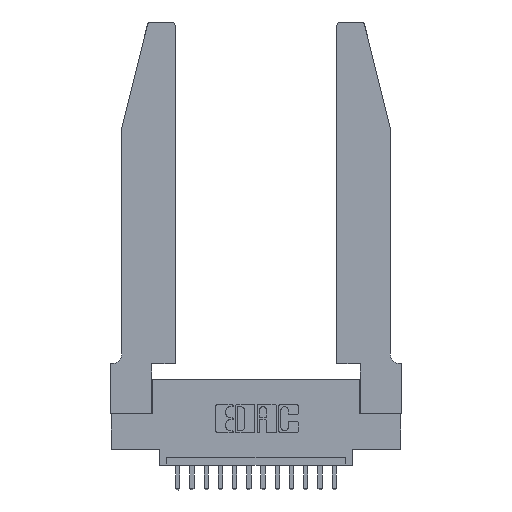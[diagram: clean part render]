
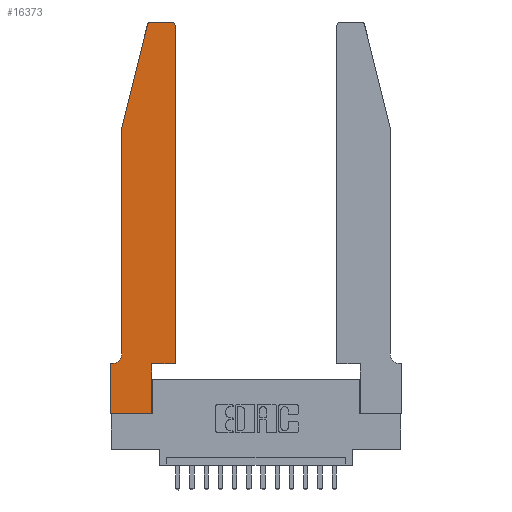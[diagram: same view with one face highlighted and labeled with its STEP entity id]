
A CAD part, top view. The second image highlights one B-rep face of the part: STEP entity #16373.
In plain terms, the highlighted planar face has unit normal (0, 0, 1).
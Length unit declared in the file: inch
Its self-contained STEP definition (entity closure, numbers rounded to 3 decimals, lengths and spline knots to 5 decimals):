
#671 = DIRECTION ( 'NONE',  ( -1., 0., 0. ) ) ;
#983 = VECTOR ( 'NONE', #1045, 39.37008 ) ;
#1045 = DIRECTION ( 'NONE',  ( 0., -1., 0. ) ) ;
#1134 = VERTEX_POINT ( 'NONE', #14228 ) ;
#1403 = CARTESIAN_POINT ( 'NONE',  ( 0.0755, 0.42, 0.37 ) ) ;
#1590 = DIRECTION ( 'NONE',  ( 1., 0., 0. ) ) ;
#1661 = VERTEX_POINT ( 'NONE', #4319 ) ;
#2010 = VERTEX_POINT ( 'NONE', #9244 ) ;
#2157 = EDGE_CURVE ( 'NONE', #10465, #15671, #2771, .T. ) ;
#2329 = ORIENTED_EDGE ( 'NONE', *, *, #8331, .T. ) ;
#2332 = AXIS2_PLACEMENT_3D ( 'NONE', #3451, #10242, #671 ) ;
#2345 = LINE ( 'NONE', #5893, #13008 ) ;
#2712 = CARTESIAN_POINT ( 'NONE',  ( 0., 0.35, 0.37 ) ) ;
#2771 = LINE ( 'NONE', #12263, #983 ) ;
#3195 = EDGE_CURVE ( 'NONE', #7690, #6580, #11854, .T. ) ;
#3210 = EDGE_CURVE ( 'NONE', #17225, #3607, #10333, .T. ) ;
#3451 = CARTESIAN_POINT ( 'NONE',  ( 0.0055, 0.42, 0.37 ) ) ;
#3607 = VERTEX_POINT ( 'NONE', #10886 ) ;
#3715 = VECTOR ( 'NONE', #16016, 39.37008 ) ;
#4100 = DIRECTION ( 'NONE',  ( 1., 0., 0. ) ) ;
#4204 = EDGE_CURVE ( 'NONE', #6601, #1134, #11837, .T. ) ;
#4209 = ORIENTED_EDGE ( 'NONE', *, *, #4634, .T. ) ;
#4242 = ORIENTED_EDGE ( 'NONE', *, *, #8408, .T. ) ;
#4319 = CARTESIAN_POINT ( 'NONE',  ( 0.25487, 2.72718, 0.37 ) ) ;
#4634 = EDGE_CURVE ( 'NONE', #15671, #6601, #13376, .T. ) ;
#4777 = CARTESIAN_POINT ( 'NONE',  ( 0., 0., 0.37 ) ) ;
#4880 = VERTEX_POINT ( 'NONE', #11902 ) ;
#5768 = VERTEX_POINT ( 'NONE', #15404 ) ;
#5893 = CARTESIAN_POINT ( 'NONE',  ( 0.0755, 2., 0.37 ) ) ;
#6005 = AXIS2_PLACEMENT_3D ( 'NONE', #2712, #12426, #4100 ) ;
#6254 = ORIENTED_EDGE ( 'NONE', *, *, #3210, .T. ) ;
#6379 = CARTESIAN_POINT ( 'NONE',  ( 0.4505, 0.35, 0.37 ) ) ;
#6580 = VERTEX_POINT ( 'NONE', #17867 ) ;
#6601 = VERTEX_POINT ( 'NONE', #16298 ) ;
#6617 = VECTOR ( 'NONE', #7564, 39.37008 ) ;
#6739 = CARTESIAN_POINT ( 'NONE',  ( 0.4505, 0.35, 0.37 ) ) ;
#6770 = CARTESIAN_POINT ( 'NONE',  ( 0.2605, 2.75, 0.37 ) ) ;
#6836 = EDGE_CURVE ( 'NONE', #4880, #5768, #14393, .T. ) ;
#6965 = DIRECTION ( 'NONE',  ( 1., 0., 0. ) ) ;
#7564 = DIRECTION ( 'NONE',  ( -1., 0., 0. ) ) ;
#7690 = VERTEX_POINT ( 'NONE', #6739 ) ;
#8027 = VECTOR ( 'NONE', #8089, 39.37008 ) ;
#8086 = EDGE_CURVE ( 'NONE', #6580, #4880, #11097, .T. ) ;
#8089 = DIRECTION ( 'NONE',  ( 1., 0., 0. ) ) ;
#8291 = ORIENTED_EDGE ( 'NONE', *, *, #16907, .T. ) ;
#8331 = EDGE_CURVE ( 'NONE', #3607, #2010, #13513, .T. ) ;
#8408 = EDGE_CURVE ( 'NONE', #5768, #1661, #16808, .T. ) ;
#8617 = VECTOR ( 'NONE', #6965, 39.37008 ) ;
#8715 = DIRECTION ( 'NONE',  ( -0.239, -0.971, 0. ) ) ;
#9244 = CARTESIAN_POINT ( 'NONE',  ( 0.2865, 0.35, 0.37 ) ) ;
#9608 = EDGE_CURVE ( 'NONE', #1134, #17225, #17212, .T. ) ;
#9738 = DIRECTION ( 'NONE',  ( -1., 0., 0. ) ) ;
#9787 = DIRECTION ( 'NONE',  ( 1., 0., 0. ) ) ;
#9829 = DIRECTION ( 'NONE',  ( 0., 1., 0. ) ) ;
#9953 = VECTOR ( 'NONE', #11041, 39.37008 ) ;
#10242 = DIRECTION ( 'NONE',  ( 0., 0., -1. ) ) ;
#10333 = LINE ( 'NONE', #16634, #8617 ) ;
#10465 = VERTEX_POINT ( 'NONE', #15127 ) ;
#10555 = EDGE_CURVE ( 'NONE', #1661, #10465, #2345, .T. ) ;
#10830 = DIRECTION ( 'NONE',  ( 0., 0., 1. ) ) ;
#10886 = CARTESIAN_POINT ( 'NONE',  ( 0.2865, 0., 0.37 ) ) ;
#10966 = VECTOR ( 'NONE', #9829, 39.37008 ) ;
#11021 = PLANE ( 'NONE',  #6005 ) ;
#11041 = DIRECTION ( 'NONE',  ( 0., -1., 0. ) ) ;
#11073 = VECTOR ( 'NONE', #9738, 39.37008 ) ;
#11094 = CARTESIAN_POINT ( 'NONE',  ( 0., 0., 0.37 ) ) ;
#11097 = CIRCLE ( 'NONE', #12567, 0.03 ) ;
#11465 = ORIENTED_EDGE ( 'NONE', *, *, #8086, .T. ) ;
#11576 = ORIENTED_EDGE ( 'NONE', *, *, #4204, .T. ) ;
#11679 = CARTESIAN_POINT ( 'NONE',  ( 0.0755, 0.35, 0.37 ) ) ;
#11837 = LINE ( 'NONE', #11679, #6617 ) ;
#11854 = LINE ( 'NONE', #14942, #10966 ) ;
#11902 = CARTESIAN_POINT ( 'NONE',  ( 0.4205, 2.75, 0.37 ) ) ;
#12164 = FACE_OUTER_BOUND ( 'NONE', #15552, .T. ) ;
#12263 = CARTESIAN_POINT ( 'NONE',  ( 0.0755, 2., 0.37 ) ) ;
#12426 = DIRECTION ( 'NONE',  ( 0., 0., 1. ) ) ;
#12567 = AXIS2_PLACEMENT_3D ( 'NONE', #15252, #10830, #1590 ) ;
#12673 = AXIS2_PLACEMENT_3D ( 'NONE', #12684, #16736, #9787 ) ;
#12684 = CARTESIAN_POINT ( 'NONE',  ( 0.284, 2.72, 0.37 ) ) ;
#12724 = ORIENTED_EDGE ( 'NONE', *, *, #10555, .T. ) ;
#13008 = VECTOR ( 'NONE', #8715, 39.37008 ) ;
#13313 = CARTESIAN_POINT ( 'NONE',  ( 0.2865, 0.35, 0.37 ) ) ;
#13376 = CIRCLE ( 'NONE', #2332, 0.07 ) ;
#13513 = LINE ( 'NONE', #13313, #3715 ) ;
#14228 = CARTESIAN_POINT ( 'NONE',  ( 0., 0.35, 0.37 ) ) ;
#14321 = ORIENTED_EDGE ( 'NONE', *, *, #3195, .T. ) ;
#14393 = LINE ( 'NONE', #6770, #11073 ) ;
#14822 = ORIENTED_EDGE ( 'NONE', *, *, #6836, .T. ) ;
#14942 = CARTESIAN_POINT ( 'NONE',  ( 0.4505, 0.35, 0.37 ) ) ;
#15127 = CARTESIAN_POINT ( 'NONE',  ( 0.0755, 2., 0.37 ) ) ;
#15252 = CARTESIAN_POINT ( 'NONE',  ( 0.4205, 2.72, 0.37 ) ) ;
#15404 = CARTESIAN_POINT ( 'NONE',  ( 0.284, 2.75, 0.37 ) ) ;
#15552 = EDGE_LOOP ( 'NONE', ( #14822, #4242, #12724, #15607, #4209, #11576, #18053, #6254, #2329, #8291, #14321, #11465 ) ) ;
#15607 = ORIENTED_EDGE ( 'NONE', *, *, #2157, .T. ) ;
#15671 = VERTEX_POINT ( 'NONE', #1403 ) ;
#16016 = DIRECTION ( 'NONE',  ( 0., 1., 0. ) ) ;
#16097 = LINE ( 'NONE', #6379, #8027 ) ;
#16298 = CARTESIAN_POINT ( 'NONE',  ( 0.0055, 0.35, 0.37 ) ) ;
#16373 = ADVANCED_FACE ( 'NONE', ( #12164 ), #11021, .T. ) ;
#16634 = CARTESIAN_POINT ( 'NONE',  ( 0., 0., 0.37 ) ) ;
#16736 = DIRECTION ( 'NONE',  ( 0., 0., 1. ) ) ;
#16808 = CIRCLE ( 'NONE', #12673, 0.03 ) ;
#16907 = EDGE_CURVE ( 'NONE', #2010, #7690, #16097, .T. ) ;
#17212 = LINE ( 'NONE', #11094, #9953 ) ;
#17225 = VERTEX_POINT ( 'NONE', #4777 ) ;
#17867 = CARTESIAN_POINT ( 'NONE',  ( 0.4505, 2.72, 0.37 ) ) ;
#18053 = ORIENTED_EDGE ( 'NONE', *, *, #9608, .T. ) ;
